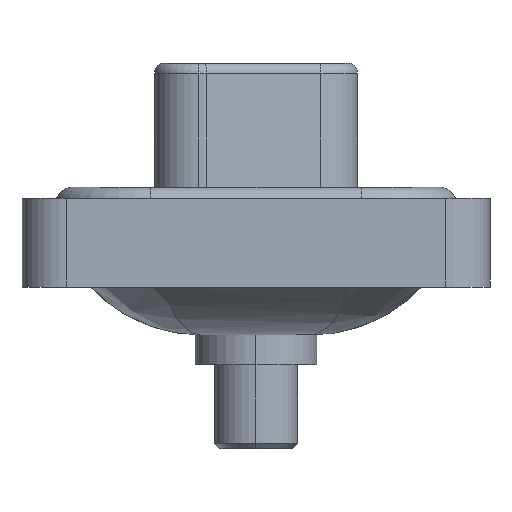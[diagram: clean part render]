
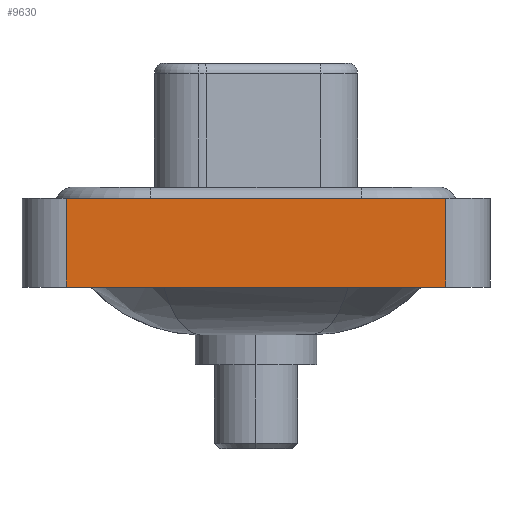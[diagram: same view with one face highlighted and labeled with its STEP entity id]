
A CAD part, left-side view. The second image highlights one B-rep face of the part: STEP entity #9630.
In plain terms, the highlighted planar face has unit normal (-1, 0, 0).
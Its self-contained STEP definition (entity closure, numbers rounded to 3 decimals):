
#79 = VECTOR ( 'NONE', #11387, 1000. ) ;
#1931 = AXIS2_PLACEMENT_3D ( 'NONE', #13276, #5080, #9779 ) ;
#2813 = LINE ( 'NONE', #7446, #7585 ) ;
#2894 = DIRECTION ( 'NONE',  ( 0., -1., 0. ) ) ;
#3250 = VERTEX_POINT ( 'NONE', #4783 ) ;
#3986 = VERTEX_POINT ( 'NONE', #5573 ) ;
#4167 = DIRECTION ( 'NONE',  ( 0., -1., 0. ) ) ;
#4176 = LINE ( 'NONE', #8808, #13316 ) ;
#4236 = CARTESIAN_POINT ( 'NONE',  ( -7.25, -8.55, 0.4 ) ) ;
#4783 = CARTESIAN_POINT ( 'NONE',  ( -7.25, 8.55, -3.6 ) ) ;
#5080 = DIRECTION ( 'NONE',  ( -1., 0., 0. ) ) ;
#5153 = VECTOR ( 'NONE', #4167, 1000. ) ;
#5272 = ORIENTED_EDGE ( 'NONE', *, *, #10262, .T. ) ;
#5573 = CARTESIAN_POINT ( 'NONE',  ( -7.25, -8.55, -3.6 ) ) ;
#5632 = VERTEX_POINT ( 'NONE', #9776 ) ;
#6044 = ORIENTED_EDGE ( 'NONE', *, *, #9156, .T. ) ;
#7446 = CARTESIAN_POINT ( 'NONE',  ( -7.25, -8.55, -3.6 ) ) ;
#7585 = VECTOR ( 'NONE', #2894, 1000. ) ;
#8112 = LINE ( 'NONE', #12599, #79 ) ;
#8808 = CARTESIAN_POINT ( 'NONE',  ( -7.25, -8.55, -3.6 ) ) ;
#9156 = EDGE_CURVE ( 'NONE', #3986, #10816, #4176, .T. ) ;
#9630 = ADVANCED_FACE ( 'NONE', ( #14341 ), #14637, .T. ) ;
#9776 = CARTESIAN_POINT ( 'NONE',  ( -7.25, 8.55, 0.4 ) ) ;
#9779 = DIRECTION ( 'NONE',  ( 0., 0., 1. ) ) ;
#10262 = EDGE_CURVE ( 'NONE', #3250, #3986, #2813, .T. ) ;
#10558 = EDGE_CURVE ( 'NONE', #3250, #5632, #8112, .T. ) ;
#10816 = VERTEX_POINT ( 'NONE', #14918 ) ;
#11387 = DIRECTION ( 'NONE',  ( 0., 0., 1. ) ) ;
#12191 = ORIENTED_EDGE ( 'NONE', *, *, #12239, .F. ) ;
#12239 = EDGE_CURVE ( 'NONE', #5632, #10816, #14787, .T. ) ;
#12599 = CARTESIAN_POINT ( 'NONE',  ( -7.25, 8.55, -3.6 ) ) ;
#13276 = CARTESIAN_POINT ( 'NONE',  ( -7.25, -8.55, -3.6 ) ) ;
#13293 = ORIENTED_EDGE ( 'NONE', *, *, #10558, .F. ) ;
#13316 = VECTOR ( 'NONE', #13437, 1000. ) ;
#13437 = DIRECTION ( 'NONE',  ( 0., 0., 1. ) ) ;
#13782 = EDGE_LOOP ( 'NONE', ( #6044, #12191, #13293, #5272 ) ) ;
#14341 = FACE_OUTER_BOUND ( 'NONE', #13782, .T. ) ;
#14637 = PLANE ( 'NONE',  #1931 ) ;
#14787 = LINE ( 'NONE', #4236, #5153 ) ;
#14918 = CARTESIAN_POINT ( 'NONE',  ( -7.25, -8.55, 0.4 ) ) ;
